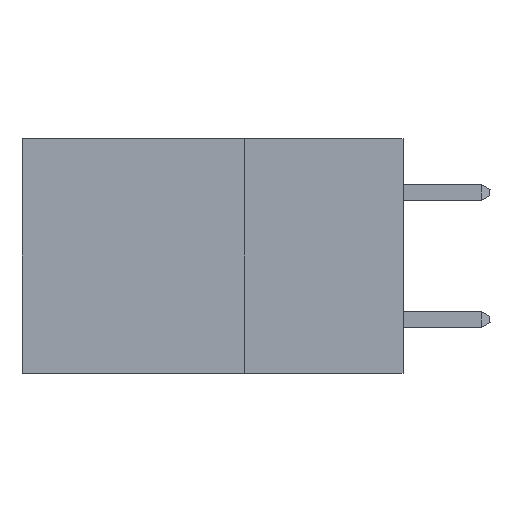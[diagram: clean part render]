
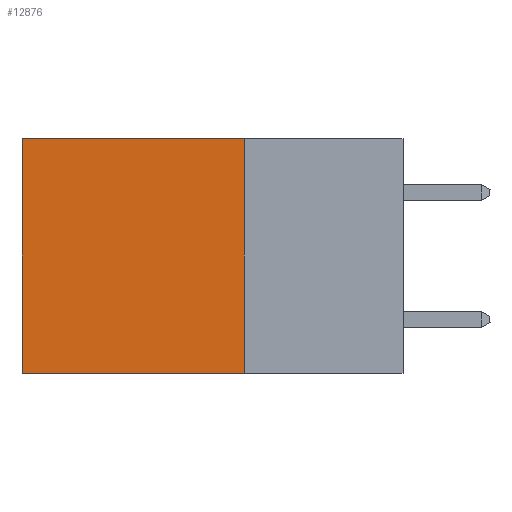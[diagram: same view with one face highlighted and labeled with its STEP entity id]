
A CAD part, left-side view. The second image highlights one B-rep face of the part: STEP entity #12876.
In plain terms, the highlighted planar face has unit normal (-1, 0, 0).
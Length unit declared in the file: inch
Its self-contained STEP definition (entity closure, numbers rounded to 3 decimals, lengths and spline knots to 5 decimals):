
#323 = CARTESIAN_POINT ( 'NONE',  ( 0.2875, 0.25, 0. ) ) ;
#3978 = VERTEX_POINT ( 'NONE', #10936 ) ;
#4339 = VERTEX_POINT ( 'NONE', #24579 ) ;
#5683 = VERTEX_POINT ( 'NONE', #32443 ) ;
#6292 = EDGE_CURVE ( 'NONE', #5683, #3978, #27194, .T. ) ;
#6391 = ORIENTED_EDGE ( 'NONE', *, *, #6292, .F. ) ;
#10936 = CARTESIAN_POINT ( 'NONE',  ( 0.2875, 0.6, -0.37 ) ) ;
#12302 = ORIENTED_EDGE ( 'NONE', *, *, #12625, .T. ) ;
#12307 = CARTESIAN_POINT ( 'NONE',  ( 0.2875, 0.25, 0. ) ) ;
#12625 = EDGE_CURVE ( 'NONE', #4339, #21416, #21534, .T. ) ;
#12876 = ADVANCED_FACE ( 'NONE', ( #33478 ), #43157, .F. ) ;
#14815 = DIRECTION ( 'NONE',  ( 0., 0., -1. ) ) ;
#20105 = LINE ( 'NONE', #323, #39013 ) ;
#20685 = EDGE_CURVE ( 'NONE', #21416, #3978, #36662, .T. ) ;
#21265 = DIRECTION ( 'NONE',  ( 1., 0., 0. ) ) ;
#21416 = VERTEX_POINT ( 'NONE', #40029 ) ;
#21534 = LINE ( 'NONE', #12307, #36925 ) ;
#24579 = CARTESIAN_POINT ( 'NONE',  ( 0.2875, 0.25, 0. ) ) ;
#27194 = LINE ( 'NONE', #27763, #38066 ) ;
#27763 = CARTESIAN_POINT ( 'NONE',  ( 0.2875, 0.25, -0.37 ) ) ;
#28118 = CARTESIAN_POINT ( 'NONE',  ( 0.2875, 0.25, 0. ) ) ;
#28469 = ORIENTED_EDGE ( 'NONE', *, *, #20685, .T. ) ;
#28573 = DIRECTION ( 'NONE',  ( 0., 0., -1. ) ) ;
#31588 = DIRECTION ( 'NONE',  ( 0., 1., 0. ) ) ;
#32441 = EDGE_CURVE ( 'NONE', #4339, #5683, #20105, .T. ) ;
#32443 = CARTESIAN_POINT ( 'NONE',  ( 0.2875, 0.25, -0.37 ) ) ;
#33478 = FACE_OUTER_BOUND ( 'NONE', #44737, .T. ) ;
#34745 = ORIENTED_EDGE ( 'NONE', *, *, #32441, .F. ) ;
#36662 = LINE ( 'NONE', #43603, #46337 ) ;
#36925 = VECTOR ( 'NONE', #37897, 39.37008 ) ;
#37897 = DIRECTION ( 'NONE',  ( 0., 1., 0. ) ) ;
#38066 = VECTOR ( 'NONE', #31588, 39.37008 ) ;
#39013 = VECTOR ( 'NONE', #14815, 39.37008 ) ;
#40029 = CARTESIAN_POINT ( 'NONE',  ( 0.2875, 0.6, 0. ) ) ;
#43157 = PLANE ( 'NONE',  #45574 ) ;
#43603 = CARTESIAN_POINT ( 'NONE',  ( 0.2875, 0.6, 0. ) ) ;
#44737 = EDGE_LOOP ( 'NONE', ( #28469, #6391, #34745, #12302 ) ) ;
#45574 = AXIS2_PLACEMENT_3D ( 'NONE', #28118, #21265, #46343 ) ;
#46337 = VECTOR ( 'NONE', #28573, 39.37008 ) ;
#46343 = DIRECTION ( 'NONE',  ( 0., 0., -1. ) ) ;
